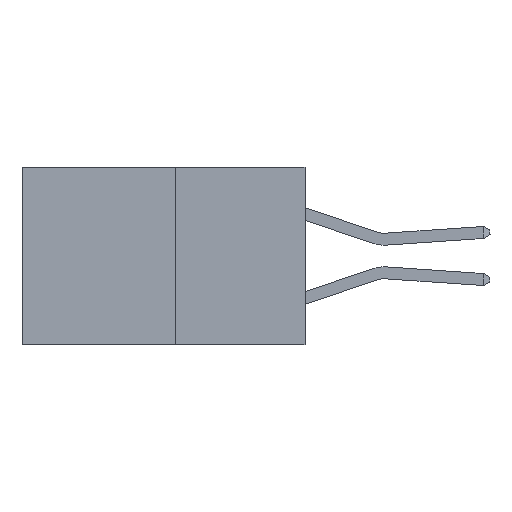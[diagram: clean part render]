
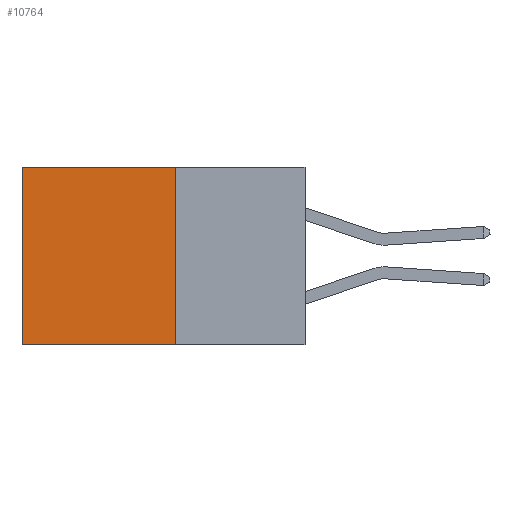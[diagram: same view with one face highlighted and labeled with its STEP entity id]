
A CAD part, left-side view. The second image highlights one B-rep face of the part: STEP entity #10764.
In plain terms, the highlighted planar face has unit normal (-1, 0, 0).
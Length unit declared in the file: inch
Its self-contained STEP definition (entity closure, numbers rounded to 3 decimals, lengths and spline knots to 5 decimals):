
#326 = DIRECTION ( 'NONE',  ( 0., 1., 0. ) ) ;
#397 = LINE ( 'NONE', #6753, #4624 ) ;
#1227 = CARTESIAN_POINT ( 'NONE',  ( 0.277, 0.59, -0.37 ) ) ;
#1853 = LINE ( 'NONE', #7269, #8836 ) ;
#1856 = EDGE_CURVE ( 'NONE', #9962, #9051, #7044, .T. ) ;
#1973 = CARTESIAN_POINT ( 'NONE',  ( 0.277, 0.27, 0. ) ) ;
#2088 = CARTESIAN_POINT ( 'NONE',  ( 0.277, 0.59, 0. ) ) ;
#2645 = ORIENTED_EDGE ( 'NONE', *, *, #12681, .F. ) ;
#3251 = EDGE_CURVE ( 'NONE', #7083, #8791, #397, .T. ) ;
#3372 = VECTOR ( 'NONE', #326, 39.37008 ) ;
#3764 = DIRECTION ( 'NONE',  ( 0., 0., -1. ) ) ;
#3921 = DIRECTION ( 'NONE',  ( 1., 0., 0. ) ) ;
#4624 = VECTOR ( 'NONE', #15001, 39.37008 ) ;
#4834 = PLANE ( 'NONE',  #9535 ) ;
#4886 = CARTESIAN_POINT ( 'NONE',  ( 0.277, 0.27, -0.37 ) ) ;
#6753 = CARTESIAN_POINT ( 'NONE',  ( 0.277, 0.27, 0. ) ) ;
#6970 = CARTESIAN_POINT ( 'NONE',  ( 0.277, 0.59, -0.37 ) ) ;
#7044 = LINE ( 'NONE', #9577, #3372 ) ;
#7073 = EDGE_LOOP ( 'NONE', ( #9427, #7133, #2645, #9045 ) ) ;
#7083 = VERTEX_POINT ( 'NONE', #1973 ) ;
#7133 = ORIENTED_EDGE ( 'NONE', *, *, #1856, .F. ) ;
#7269 = CARTESIAN_POINT ( 'NONE',  ( 0.277, 0.27, -0.37 ) ) ;
#7830 = FACE_OUTER_BOUND ( 'NONE', #7073, .T. ) ;
#8791 = VERTEX_POINT ( 'NONE', #2088 ) ;
#8836 = VECTOR ( 'NONE', #16753, 39.37008 ) ;
#9045 = ORIENTED_EDGE ( 'NONE', *, *, #3251, .T. ) ;
#9051 = VERTEX_POINT ( 'NONE', #1227 ) ;
#9120 = CARTESIAN_POINT ( 'NONE',  ( 0.277, 0.27, -0.37 ) ) ;
#9427 = ORIENTED_EDGE ( 'NONE', *, *, #17042, .T. ) ;
#9535 = AXIS2_PLACEMENT_3D ( 'NONE', #4886, #3921, #3764 ) ;
#9577 = CARTESIAN_POINT ( 'NONE',  ( 0.277, 0.27, -0.37 ) ) ;
#9962 = VERTEX_POINT ( 'NONE', #9120 ) ;
#10764 = ADVANCED_FACE ( 'NONE', ( #7830 ), #4834, .F. ) ;
#11328 = VECTOR ( 'NONE', #12405, 39.37008 ) ;
#12405 = DIRECTION ( 'NONE',  ( 0., 0., -1. ) ) ;
#12681 = EDGE_CURVE ( 'NONE', #7083, #9962, #1853, .T. ) ;
#14899 = LINE ( 'NONE', #6970, #11328 ) ;
#15001 = DIRECTION ( 'NONE',  ( 0., 1., 0. ) ) ;
#16753 = DIRECTION ( 'NONE',  ( 0., 0., -1. ) ) ;
#17042 = EDGE_CURVE ( 'NONE', #8791, #9051, #14899, .T. ) ;
